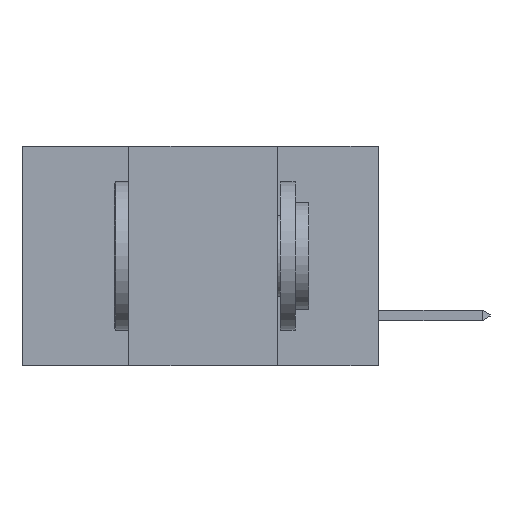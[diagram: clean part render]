
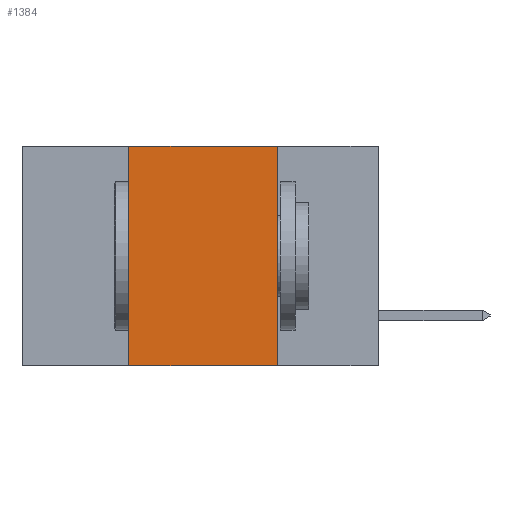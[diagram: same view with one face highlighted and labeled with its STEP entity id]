
A CAD part, left-side view. The second image highlights one B-rep face of the part: STEP entity #1384.
In plain terms, the highlighted planar face has unit normal (-1, 0, 0).
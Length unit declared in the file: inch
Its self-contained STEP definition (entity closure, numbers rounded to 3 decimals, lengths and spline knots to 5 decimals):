
#157 = LINE ( 'NONE', #8729, #5051 ) ;
#325 = DIRECTION ( 'NONE',  ( 0., 0., -1. ) ) ;
#513 = CARTESIAN_POINT ( 'NONE',  ( 0., 0.17, 0. ) ) ;
#1384 = ADVANCED_FACE ( 'NONE', ( #3900 ), #2123, .F. ) ;
#1536 = VERTEX_POINT ( 'NONE', #11827 ) ;
#1810 = AXIS2_PLACEMENT_3D ( 'NONE', #4263, #4967, #325 ) ;
#2123 = PLANE ( 'NONE',  #1810 ) ;
#3080 = ORIENTED_EDGE ( 'NONE', *, *, #3819, .T. ) ;
#3095 = ORIENTED_EDGE ( 'NONE', *, *, #3192, .F. ) ;
#3143 = CARTESIAN_POINT ( 'NONE',  ( 0., 0.42, -0.37 ) ) ;
#3153 = ORIENTED_EDGE ( 'NONE', *, *, #12024, .F. ) ;
#3163 = ORIENTED_EDGE ( 'NONE', *, *, #11431, .F. ) ;
#3192 = EDGE_CURVE ( 'NONE', #6144, #1536, #7442, .T. ) ;
#3234 = DIRECTION ( 'NONE',  ( 0., 0., -1. ) ) ;
#3444 = VECTOR ( 'NONE', #3234, 39.37008 ) ;
#3577 = VECTOR ( 'NONE', #8414, 39.37008 ) ;
#3819 = EDGE_CURVE ( 'NONE', #6144, #5447, #157, .T. ) ;
#3900 = FACE_OUTER_BOUND ( 'NONE', #9812, .T. ) ;
#3980 = CARTESIAN_POINT ( 'NONE',  ( 0., 0.17, -0.37 ) ) ;
#4263 = CARTESIAN_POINT ( 'NONE',  ( 0., 0.6, 0. ) ) ;
#4627 = VECTOR ( 'NONE', #6700, 39.37008 ) ;
#4631 = VERTEX_POINT ( 'NONE', #513 ) ;
#4967 = DIRECTION ( 'NONE',  ( 1., 0., 0. ) ) ;
#5051 = VECTOR ( 'NONE', #9196, 39.37008 ) ;
#5447 = VERTEX_POINT ( 'NONE', #3980 ) ;
#6115 = LINE ( 'NONE', #7496, #3577 ) ;
#6144 = VERTEX_POINT ( 'NONE', #3143 ) ;
#6304 = CARTESIAN_POINT ( 'NONE',  ( 0., 0.42, -0.37 ) ) ;
#6700 = DIRECTION ( 'NONE',  ( 0., 0., 1. ) ) ;
#7442 = LINE ( 'NONE', #6304, #4627 ) ;
#7496 = CARTESIAN_POINT ( 'NONE',  ( 0., 0.6, 0. ) ) ;
#8414 = DIRECTION ( 'NONE',  ( 0., -1., 0. ) ) ;
#8729 = CARTESIAN_POINT ( 'NONE',  ( 0., 0.6, -0.37 ) ) ;
#8816 = CARTESIAN_POINT ( 'NONE',  ( 0., 0.17, -0.37 ) ) ;
#9196 = DIRECTION ( 'NONE',  ( 0., -1., 0. ) ) ;
#9812 = EDGE_LOOP ( 'NONE', ( #3163, #3153, #3095, #3080 ) ) ;
#10246 = LINE ( 'NONE', #8816, #3444 ) ;
#11431 = EDGE_CURVE ( 'NONE', #4631, #5447, #10246, .T. ) ;
#11827 = CARTESIAN_POINT ( 'NONE',  ( 0., 0.42, 0. ) ) ;
#12024 = EDGE_CURVE ( 'NONE', #1536, #4631, #6115, .T. ) ;
